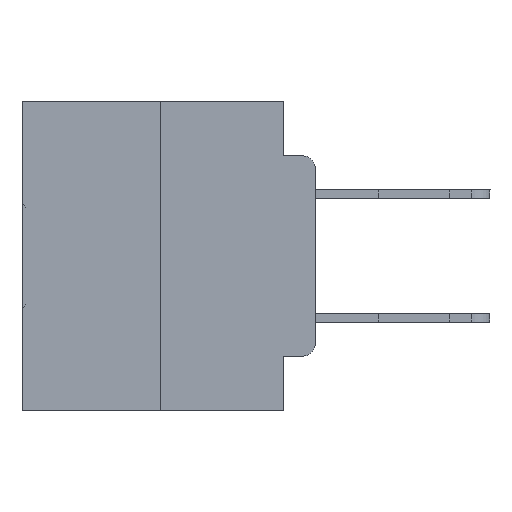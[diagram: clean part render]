
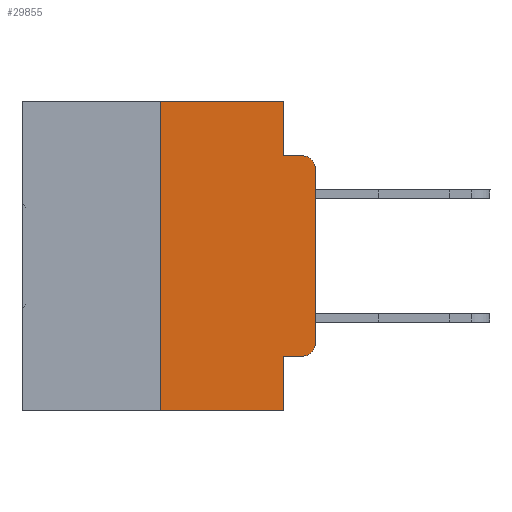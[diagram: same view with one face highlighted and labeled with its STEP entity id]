
A CAD part, left-side view. The second image highlights one B-rep face of the part: STEP entity #29855.
In plain terms, the highlighted planar face has unit normal (-1, 0, 0).
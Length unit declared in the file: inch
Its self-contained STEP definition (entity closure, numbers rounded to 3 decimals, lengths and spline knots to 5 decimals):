
#462 = DIRECTION ( 'NONE',  ( 1., 0., 0. ) ) ;
#545 = VERTEX_POINT ( 'NONE', #26716 ) ;
#701 = ORIENTED_EDGE ( 'NONE', *, *, #13362, .F. ) ;
#811 = CARTESIAN_POINT ( 'NONE',  ( 0., 0.051, -0.0885 ) ) ;
#1252 = ORIENTED_EDGE ( 'NONE', *, *, #6271, .T. ) ;
#1273 = VECTOR ( 'NONE', #26126, 39.37008 ) ;
#1698 = VECTOR ( 'NONE', #23621, 39.37008 ) ;
#2014 = CARTESIAN_POINT ( 'NONE',  ( 0., 0.02, -0.1085 ) ) ;
#3515 = LINE ( 'NONE', #28063, #17936 ) ;
#3636 = EDGE_LOOP ( 'NONE', ( #16817, #7181, #24887, #701, #33007, #13812, #1252, #12309, #28480, #18236 ) ) ;
#3755 = CARTESIAN_POINT ( 'NONE',  ( 0., 0.051, -0.4115 ) ) ;
#3843 = CARTESIAN_POINT ( 'NONE',  ( 0., 0.051, -0.0885 ) ) ;
#4996 = VERTEX_POINT ( 'NONE', #27039 ) ;
#5307 = EDGE_CURVE ( 'NONE', #6973, #545, #32099, .T. ) ;
#5410 = VERTEX_POINT ( 'NONE', #3843 ) ;
#5579 = DIRECTION ( 'NONE',  ( 0., 0., -1. ) ) ;
#6271 = EDGE_CURVE ( 'NONE', #17607, #14837, #14851, .T. ) ;
#6973 = VERTEX_POINT ( 'NONE', #27917 ) ;
#7129 = CARTESIAN_POINT ( 'NONE',  ( 0., 0.473, -0.5 ) ) ;
#7181 = ORIENTED_EDGE ( 'NONE', *, *, #31611, .T. ) ;
#7453 = LINE ( 'NONE', #21438, #20276 ) ;
#8055 = VERTEX_POINT ( 'NONE', #21244 ) ;
#8120 = DIRECTION ( 'NONE',  ( 0., 0., 1. ) ) ;
#8260 = VECTOR ( 'NONE', #28387, 39.37008 ) ;
#8833 = AXIS2_PLACEMENT_3D ( 'NONE', #2014, #20239, #12422 ) ;
#9832 = DIRECTION ( 'NONE',  ( 0., 0., 1. ) ) ;
#10167 = VERTEX_POINT ( 'NONE', #28604 ) ;
#10471 = VECTOR ( 'NONE', #11992, 39.37008 ) ;
#10590 = DIRECTION ( 'NONE',  ( 0., 0., -1. ) ) ;
#10692 = EDGE_CURVE ( 'NONE', #5410, #10167, #27710, .T. ) ;
#11097 = PLANE ( 'NONE',  #29362 ) ;
#11262 = CARTESIAN_POINT ( 'NONE',  ( 0., 0.473, 0. ) ) ;
#11992 = DIRECTION ( 'NONE',  ( 0., -1., 0. ) ) ;
#12309 = ORIENTED_EDGE ( 'NONE', *, *, #28646, .F. ) ;
#12422 = DIRECTION ( 'NONE',  ( 0., 0., -1. ) ) ;
#13362 = EDGE_CURVE ( 'NONE', #545, #5410, #23923, .T. ) ;
#13687 = FACE_OUTER_BOUND ( 'NONE', #3636, .T. ) ;
#13812 = ORIENTED_EDGE ( 'NONE', *, *, #18416, .F. ) ;
#13954 = EDGE_CURVE ( 'NONE', #30620, #32012, #27873, .T. ) ;
#14837 = VERTEX_POINT ( 'NONE', #16258 ) ;
#14851 = LINE ( 'NONE', #7129, #10471 ) ;
#15013 = VECTOR ( 'NONE', #30359, 39.37008 ) ;
#16258 = CARTESIAN_POINT ( 'NONE',  ( 0., 0.051, -0.5 ) ) ;
#16603 = LINE ( 'NONE', #32822, #15013 ) ;
#16817 = ORIENTED_EDGE ( 'NONE', *, *, #19242, .T. ) ;
#17136 = VECTOR ( 'NONE', #18345, 39.37008 ) ;
#17607 = VERTEX_POINT ( 'NONE', #32371 ) ;
#17936 = VECTOR ( 'NONE', #9832, 39.37008 ) ;
#18236 = ORIENTED_EDGE ( 'NONE', *, *, #25249, .T. ) ;
#18317 = CARTESIAN_POINT ( 'NONE',  ( 0., 0.051, -0.4115 ) ) ;
#18345 = DIRECTION ( 'NONE',  ( 0., 0., -1. ) ) ;
#18416 = EDGE_CURVE ( 'NONE', #17607, #6973, #3515, .T. ) ;
#19242 = EDGE_CURVE ( 'NONE', #8055, #4996, #7453, .T. ) ;
#20135 = CARTESIAN_POINT ( 'NONE',  ( 0., 0.051, 0. ) ) ;
#20239 = DIRECTION ( 'NONE',  ( -1., 0., 0. ) ) ;
#20276 = VECTOR ( 'NONE', #8120, 39.37008 ) ;
#21244 = CARTESIAN_POINT ( 'NONE',  ( 0., 0., -0.3915 ) ) ;
#21438 = CARTESIAN_POINT ( 'NONE',  ( 0., 0., 0. ) ) ;
#23114 = DIRECTION ( 'NONE',  ( -1., 0., 0. ) ) ;
#23621 = DIRECTION ( 'NONE',  ( 0., -1., 0. ) ) ;
#23923 = LINE ( 'NONE', #20135, #17136 ) ;
#24887 = ORIENTED_EDGE ( 'NONE', *, *, #10692, .F. ) ;
#25249 = EDGE_CURVE ( 'NONE', #32012, #8055, #28444, .T. ) ;
#26126 = DIRECTION ( 'NONE',  ( 0., -1., 0. ) ) ;
#26716 = CARTESIAN_POINT ( 'NONE',  ( 0., 0.051, 0. ) ) ;
#27039 = CARTESIAN_POINT ( 'NONE',  ( 0., 0., -0.1085 ) ) ;
#27710 = LINE ( 'NONE', #811, #1698 ) ;
#27873 = LINE ( 'NONE', #18317, #8260 ) ;
#27917 = CARTESIAN_POINT ( 'NONE',  ( 0., 0.25, 0. ) ) ;
#28063 = CARTESIAN_POINT ( 'NONE',  ( 0., 0.25, 0. ) ) ;
#28387 = DIRECTION ( 'NONE',  ( 0., -1., 0. ) ) ;
#28444 = CIRCLE ( 'NONE', #28835, 0.02 ) ;
#28480 = ORIENTED_EDGE ( 'NONE', *, *, #13954, .T. ) ;
#28604 = CARTESIAN_POINT ( 'NONE',  ( 0., 0.02, -0.0885 ) ) ;
#28646 = EDGE_CURVE ( 'NONE', #30620, #14837, #16603, .T. ) ;
#28835 = AXIS2_PLACEMENT_3D ( 'NONE', #30723, #23114, #10590 ) ;
#29362 = AXIS2_PLACEMENT_3D ( 'NONE', #31452, #462, #5579 ) ;
#29855 = ADVANCED_FACE ( 'NONE', ( #13687 ), #11097, .F. ) ;
#30030 = CIRCLE ( 'NONE', #8833, 0.02 ) ;
#30359 = DIRECTION ( 'NONE',  ( 0., 0., -1. ) ) ;
#30620 = VERTEX_POINT ( 'NONE', #3755 ) ;
#30723 = CARTESIAN_POINT ( 'NONE',  ( 0., 0.02, -0.3915 ) ) ;
#31452 = CARTESIAN_POINT ( 'NONE',  ( 0., 0.473, 0. ) ) ;
#31611 = EDGE_CURVE ( 'NONE', #4996, #10167, #30030, .T. ) ;
#31766 = CARTESIAN_POINT ( 'NONE',  ( 0., 0.02, -0.4115 ) ) ;
#32012 = VERTEX_POINT ( 'NONE', #31766 ) ;
#32099 = LINE ( 'NONE', #11262, #1273 ) ;
#32371 = CARTESIAN_POINT ( 'NONE',  ( 0., 0.25, -0.5 ) ) ;
#32822 = CARTESIAN_POINT ( 'NONE',  ( 0., 0.051, 0. ) ) ;
#33007 = ORIENTED_EDGE ( 'NONE', *, *, #5307, .F. ) ;
